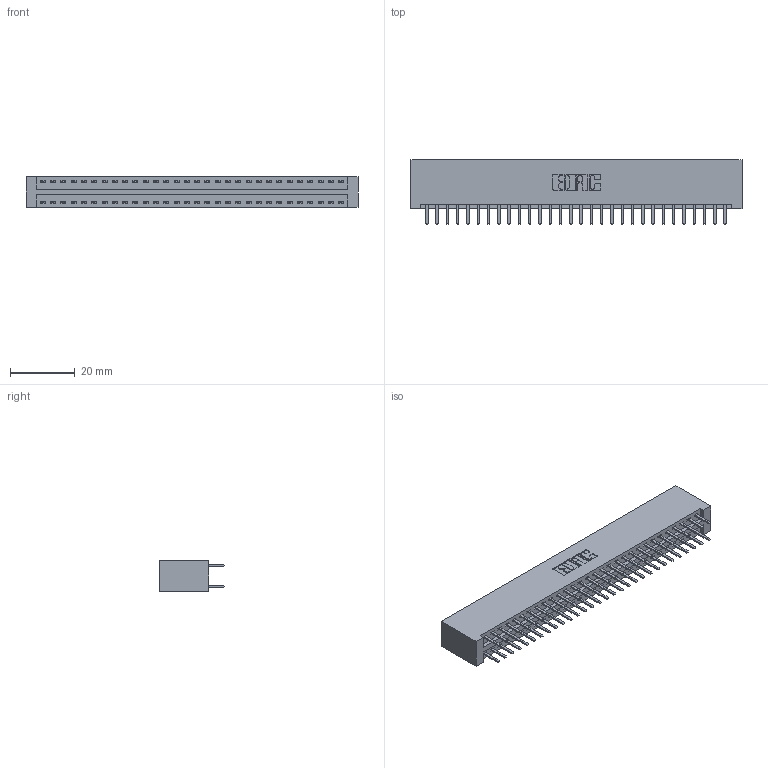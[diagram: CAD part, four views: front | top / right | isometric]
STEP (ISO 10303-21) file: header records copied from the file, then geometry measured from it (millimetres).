
FILE_DESCRIPTION (( 'STEP AP203' ), '1' );
FILE_NAME ('346-060-520-201.STEP', '2022-05-21T10:16:09', ( '' ), ( '' ), 'SwSTEP 2.0', 'SolidWorks 2020', '' );
FILE_SCHEMA (( 'CONFIG_CONTROL_DESIGN' ));
Length unit declared in the file: inch
Products named in the file (3): 346 Part_No Mounting Lugs; 345-292-001_345-293-120; 346-060-520-201
Assembly tree (61 placements, depth 2):
  346-060-520-201
    346 Part_No Mounting Lugs
    345-292-001_345-293-120  x60
Bounding box: 102.49 x 20.02 x 9.4 mm (x, y, z)
Volume: 10447.7 mm3; surface area: 14273.8 mm2
Topology: 61 solids, 61 shells, 3474 faces, 10085 edges, 6562 vertices
Faces by surface type: plane 2292, cylinder 1182
Entity records: 21031 total; most frequent: CARTESIAN_POINT 3492, ORIENTED_EDGE 3414, DIRECTION 3111, EDGE_CURVE 1707, VECTOR 1459, LINE 1459, VERTEX_POINT 1134, AXIS2_PLACEMENT_3D 826
